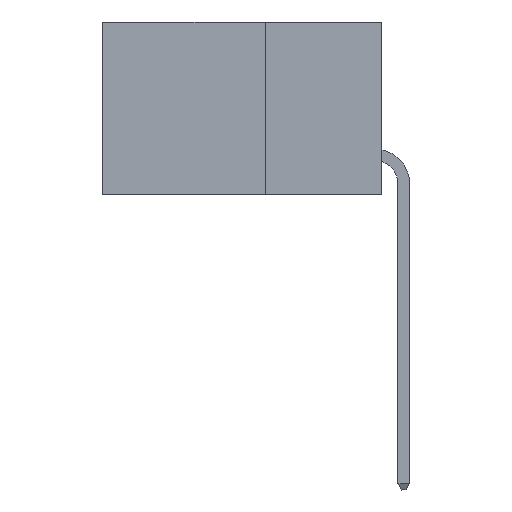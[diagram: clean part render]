
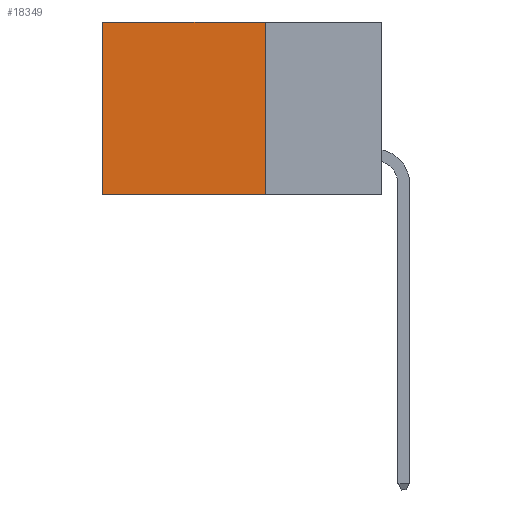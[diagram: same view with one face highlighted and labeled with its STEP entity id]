
A CAD part, left-side view. The second image highlights one B-rep face of the part: STEP entity #18349.
In plain terms, the highlighted planar face has unit normal (-1, 0, 0).
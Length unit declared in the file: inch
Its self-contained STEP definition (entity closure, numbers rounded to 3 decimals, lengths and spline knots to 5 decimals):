
#303 = VERTEX_POINT ( 'NONE', #7031 ) ;
#5905 = CARTESIAN_POINT ( 'NONE',  ( 0.2875, 0.6, 0. ) ) ;
#6933 = CARTESIAN_POINT ( 'NONE',  ( 0.2875, 0.6, -0.37 ) ) ;
#7031 = CARTESIAN_POINT ( 'NONE',  ( 0.2875, 0.6, 0. ) ) ;
#8603 = VECTOR ( 'NONE', #24963, 39.37008 ) ;
#9657 = CARTESIAN_POINT ( 'NONE',  ( 0.2875, 0.25, -0.37 ) ) ;
#11230 = VERTEX_POINT ( 'NONE', #38682 ) ;
#11666 = AXIS2_PLACEMENT_3D ( 'NONE', #18869, #41406, #22158 ) ;
#12851 = EDGE_CURVE ( 'NONE', #33280, #28382, #25349, .T. ) ;
#14609 = CARTESIAN_POINT ( 'NONE',  ( 0.2875, 0.25, 0. ) ) ;
#16654 = VECTOR ( 'NONE', #22804, 39.37008 ) ;
#16853 = FACE_OUTER_BOUND ( 'NONE', #18638, .T. ) ;
#17245 = EDGE_CURVE ( 'NONE', #303, #28382, #33088, .T. ) ;
#18349 = ADVANCED_FACE ( 'NONE', ( #16853 ), #38229, .F. ) ;
#18395 = CARTESIAN_POINT ( 'NONE',  ( 0.2875, 0.25, 0. ) ) ;
#18638 = EDGE_LOOP ( 'NONE', ( #30523, #19174, #41557, #36784 ) ) ;
#18869 = CARTESIAN_POINT ( 'NONE',  ( 0.2875, 0.25, 0. ) ) ;
#19174 = ORIENTED_EDGE ( 'NONE', *, *, #12851, .F. ) ;
#22070 = DIRECTION ( 'NONE',  ( 0., 0., -1. ) ) ;
#22158 = DIRECTION ( 'NONE',  ( 0., 0., -1. ) ) ;
#22673 = VECTOR ( 'NONE', #24340, 39.37008 ) ;
#22804 = DIRECTION ( 'NONE',  ( 0., 1., 0. ) ) ;
#24340 = DIRECTION ( 'NONE',  ( 0., 1., 0. ) ) ;
#24963 = DIRECTION ( 'NONE',  ( 0., 0., -1. ) ) ;
#25349 = LINE ( 'NONE', #9657, #16654 ) ;
#28382 = VERTEX_POINT ( 'NONE', #6933 ) ;
#29856 = EDGE_CURVE ( 'NONE', #11230, #33280, #34551, .T. ) ;
#30523 = ORIENTED_EDGE ( 'NONE', *, *, #17245, .T. ) ;
#33088 = LINE ( 'NONE', #5905, #41569 ) ;
#33280 = VERTEX_POINT ( 'NONE', #33304 ) ;
#33304 = CARTESIAN_POINT ( 'NONE',  ( 0.2875, 0.25, -0.37 ) ) ;
#34551 = LINE ( 'NONE', #18395, #8603 ) ;
#36784 = ORIENTED_EDGE ( 'NONE', *, *, #41163, .T. ) ;
#38229 = PLANE ( 'NONE',  #11666 ) ;
#38682 = CARTESIAN_POINT ( 'NONE',  ( 0.2875, 0.25, 0. ) ) ;
#39777 = LINE ( 'NONE', #14609, #22673 ) ;
#41163 = EDGE_CURVE ( 'NONE', #11230, #303, #39777, .T. ) ;
#41406 = DIRECTION ( 'NONE',  ( 1., 0., 0. ) ) ;
#41557 = ORIENTED_EDGE ( 'NONE', *, *, #29856, .F. ) ;
#41569 = VECTOR ( 'NONE', #22070, 39.37008 ) ;
